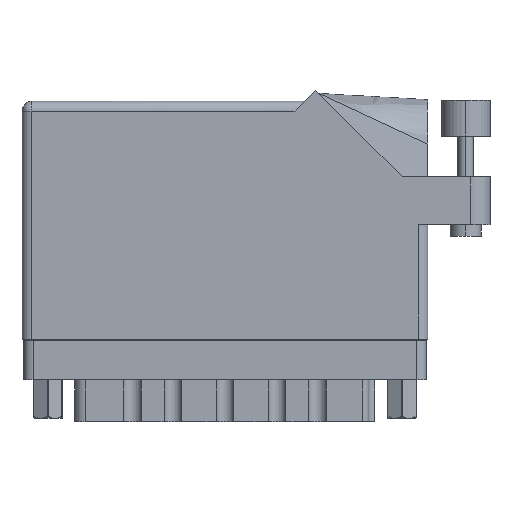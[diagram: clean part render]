
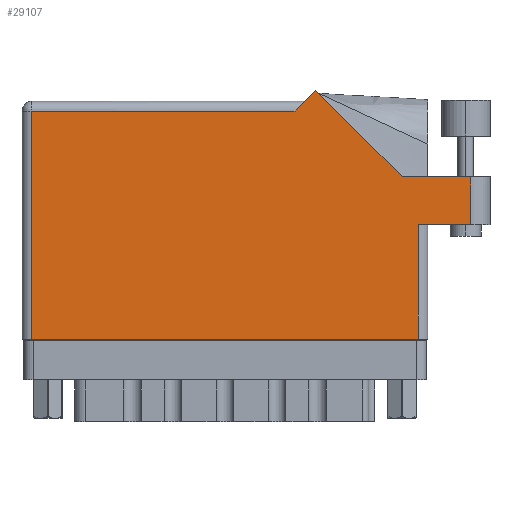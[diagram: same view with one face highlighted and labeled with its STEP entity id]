
A CAD part, front view. The second image highlights one B-rep face of the part: STEP entity #29107.
In plain terms, the highlighted face is planar.
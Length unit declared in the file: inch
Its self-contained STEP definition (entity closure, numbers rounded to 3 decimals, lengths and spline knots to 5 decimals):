
#825 = CARTESIAN_POINT ( 'NONE',  ( 2.612, 0.737, 0. ) ) ;
#1028 = LINE ( 'NONE', #825, #27616 ) ;
#1150 = VERTEX_POINT ( 'NONE', #1386 ) ;
#1238 = LINE ( 'NONE', #30069, #50112 ) ;
#1260 = DIRECTION ( 'NONE',  ( 0., 0., -1. ) ) ;
#1310 = LINE ( 'NONE', #15772, #22281 ) ;
#1386 = CARTESIAN_POINT ( 'NONE',  ( 2.44642, 1.044, 0. ) ) ;
#2402 = CARTESIAN_POINT ( 'NONE',  ( 2.887, 0.737, 0. ) ) ;
#3035 = VECTOR ( 'NONE', #8078, 39.37008 ) ;
#3541 = CARTESIAN_POINT ( 'NONE',  ( 0., 1.468, 0. ) ) ;
#4369 = AXIS2_PLACEMENT_3D ( 'NONE', #41309, #1260, #32530 ) ;
#4874 = EDGE_CURVE ( 'NONE', #14111, #8375, #1028, .T. ) ;
#6560 = DIRECTION ( 'NONE',  ( -0.707, 0.707, 0. ) ) ;
#8078 = DIRECTION ( 'NONE',  ( -1., 0., 0. ) ) ;
#8375 = VERTEX_POINT ( 'NONE', #2402 ) ;
#8386 = CARTESIAN_POINT ( 'NONE',  ( 2.55, 0.737, 0. ) ) ;
#8984 = ORIENTED_EDGE ( 'NONE', *, *, #20958, .T. ) ;
#10050 = EDGE_CURVE ( 'NONE', #52229, #14111, #15059, .T. ) ;
#10276 = DIRECTION ( 'NONE',  ( 0., 1., 0. ) ) ;
#10623 = CARTESIAN_POINT ( 'NONE',  ( 2.55, 0., 0. ) ) ;
#10874 = PLANE ( 'NONE',  #4369 ) ;
#13074 = DIRECTION ( 'NONE',  ( 0., -1., 0. ) ) ;
#14111 = VERTEX_POINT ( 'NONE', #8386 ) ;
#15059 = LINE ( 'NONE', #35972, #24784 ) ;
#15257 = CARTESIAN_POINT ( 'NONE',  ( 3.012, 1.044, 0. ) ) ;
#15772 = CARTESIAN_POINT ( 'NONE',  ( 0., 0., 0. ) ) ;
#16572 = LINE ( 'NONE', #49997, #46523 ) ;
#18010 = EDGE_CURVE ( 'NONE', #56154, #35219, #1238, .T. ) ;
#18525 = EDGE_CURVE ( 'NONE', #46655, #52229, #1310, .T. ) ;
#20958 = EDGE_CURVE ( 'NONE', #8375, #22405, #16572, .T. ) ;
#21599 = VECTOR ( 'NONE', #50297, 39.37008 ) ;
#22047 = ORIENTED_EDGE ( 'NONE', *, *, #23509, .T. ) ;
#22281 = VECTOR ( 'NONE', #42294, 39.37008 ) ;
#22405 = VERTEX_POINT ( 'NONE', #42944 ) ;
#23509 = EDGE_CURVE ( 'NONE', #1150, #56154, #48261, .T. ) ;
#24784 = VECTOR ( 'NONE', #40461, 39.37008 ) ;
#27616 = VECTOR ( 'NONE', #36005, 39.37008 ) ;
#28899 = ORIENTED_EDGE ( 'NONE', *, *, #10050, .T. ) ;
#29107 = ADVANCED_FACE ( 'NONE', ( #40888 ), #10874, .F. ) ;
#30069 = CARTESIAN_POINT ( 'NONE',  ( 1.819, 1.53, 0. ) ) ;
#30514 = ORIENTED_EDGE ( 'NONE', *, *, #50142, .T. ) ;
#32530 = DIRECTION ( 'NONE',  ( -1., 0., 0. ) ) ;
#32740 = ORIENTED_EDGE ( 'NONE', *, *, #18010, .T. ) ;
#33494 = EDGE_LOOP ( 'NONE', ( #47274, #8984, #43347, #22047, #32740, #30514, #55216, #35135, #28899 ) ) ;
#34743 = CARTESIAN_POINT ( 'NONE',  ( 0.062, 0., 0. ) ) ;
#35135 = ORIENTED_EDGE ( 'NONE', *, *, #18525, .T. ) ;
#35219 = VERTEX_POINT ( 'NONE', #49899 ) ;
#35972 = CARTESIAN_POINT ( 'NONE',  ( 2.55, 0.737, 0. ) ) ;
#36005 = DIRECTION ( 'NONE',  ( 1., 0., 0. ) ) ;
#37167 = VECTOR ( 'NONE', #6560, 39.37008 ) ;
#38633 = DIRECTION ( 'NONE',  ( -0.707, -0.707, 0. ) ) ;
#38935 = EDGE_CURVE ( 'NONE', #52662, #46655, #40920, .T. ) ;
#39500 = VECTOR ( 'NONE', #13074, 39.37008 ) ;
#39821 = CARTESIAN_POINT ( 'NONE',  ( 0.062, 0., 0. ) ) ;
#40461 = DIRECTION ( 'NONE',  ( 0., 1., 0. ) ) ;
#40888 = FACE_OUTER_BOUND ( 'NONE', #33494, .T. ) ;
#40920 = LINE ( 'NONE', #39821, #39500 ) ;
#40986 = CARTESIAN_POINT ( 'NONE',  ( 1.88971, 1.60071, 0. ) ) ;
#41309 = CARTESIAN_POINT ( 'NONE',  ( 0., 1.53, 0. ) ) ;
#42294 = DIRECTION ( 'NONE',  ( 1., 0., 0. ) ) ;
#42534 = LINE ( 'NONE', #15257, #21599 ) ;
#42944 = CARTESIAN_POINT ( 'NONE',  ( 2.887, 1.044, 0. ) ) ;
#43347 = ORIENTED_EDGE ( 'NONE', *, *, #54185, .T. ) ;
#43569 = LINE ( 'NONE', #3541, #3035 ) ;
#46523 = VECTOR ( 'NONE', #10276, 39.37008 ) ;
#46655 = VERTEX_POINT ( 'NONE', #34743 ) ;
#47274 = ORIENTED_EDGE ( 'NONE', *, *, #4874, .T. ) ;
#48261 = LINE ( 'NONE', #55650, #37167 ) ;
#49302 = CARTESIAN_POINT ( 'NONE',  ( 0.062, 1.468, 0. ) ) ;
#49899 = CARTESIAN_POINT ( 'NONE',  ( 1.757, 1.468, 0. ) ) ;
#49997 = CARTESIAN_POINT ( 'NONE',  ( 2.887, 1.044, 0. ) ) ;
#50112 = VECTOR ( 'NONE', #38633, 39.37008 ) ;
#50142 = EDGE_CURVE ( 'NONE', #35219, #52662, #43569, .T. ) ;
#50297 = DIRECTION ( 'NONE',  ( -1., 0., 0. ) ) ;
#52229 = VERTEX_POINT ( 'NONE', #10623 ) ;
#52662 = VERTEX_POINT ( 'NONE', #49302 ) ;
#54185 = EDGE_CURVE ( 'NONE', #22405, #1150, #42534, .T. ) ;
#55216 = ORIENTED_EDGE ( 'NONE', *, *, #38935, .T. ) ;
#55650 = CARTESIAN_POINT ( 'NONE',  ( 2.44642, 1.044, 0. ) ) ;
#56154 = VERTEX_POINT ( 'NONE', #40986 ) ;
